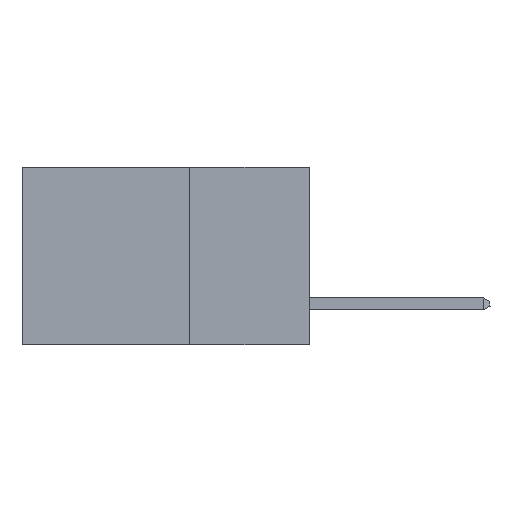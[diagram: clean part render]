
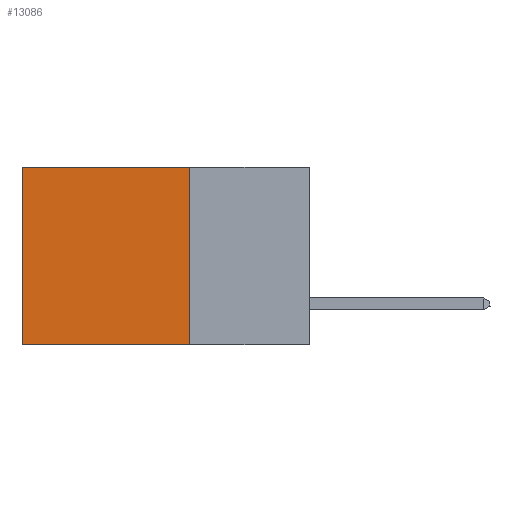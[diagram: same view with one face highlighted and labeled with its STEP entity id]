
A CAD part, left-side view. The second image highlights one B-rep face of the part: STEP entity #13086.
In plain terms, the highlighted planar face has unit normal (-1, 0, 0).
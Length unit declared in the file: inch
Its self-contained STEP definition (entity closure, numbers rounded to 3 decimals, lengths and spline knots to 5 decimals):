
#238 = VERTEX_POINT ( 'NONE', #27249 ) ;
#965 = CARTESIAN_POINT ( 'NONE',  ( 0.2875, 0.25, -0.37 ) ) ;
#1485 = VERTEX_POINT ( 'NONE', #13340 ) ;
#1870 = FACE_OUTER_BOUND ( 'NONE', #26713, .T. ) ;
#3059 = PLANE ( 'NONE',  #14644 ) ;
#4616 = LINE ( 'NONE', #22239, #10946 ) ;
#7609 = DIRECTION ( 'NONE',  ( 0., 1., 0. ) ) ;
#8184 = CARTESIAN_POINT ( 'NONE',  ( 0.2875, 0.6, -0.37 ) ) ;
#8716 = EDGE_CURVE ( 'NONE', #238, #26380, #4616, .T. ) ;
#10644 = CARTESIAN_POINT ( 'NONE',  ( 0.2875, 0.25, -0.37 ) ) ;
#10946 = VECTOR ( 'NONE', #24400, 39.37008 ) ;
#12156 = VECTOR ( 'NONE', #7609, 39.37008 ) ;
#13086 = ADVANCED_FACE ( 'NONE', ( #1870 ), #3059, .F. ) ;
#13340 = CARTESIAN_POINT ( 'NONE',  ( 0.2875, 0.6, 0. ) ) ;
#14644 = AXIS2_PLACEMENT_3D ( 'NONE', #20826, #16453, #18583 ) ;
#16453 = DIRECTION ( 'NONE',  ( 1., 0., 0. ) ) ;
#16570 = EDGE_CURVE ( 'NONE', #238, #1485, #28032, .T. ) ;
#16613 = EDGE_CURVE ( 'NONE', #1485, #22886, #25552, .T. ) ;
#17371 = DIRECTION ( 'NONE',  ( 0., 0., -1. ) ) ;
#17514 = VECTOR ( 'NONE', #28062, 39.37008 ) ;
#18132 = LINE ( 'NONE', #965, #12156 ) ;
#18583 = DIRECTION ( 'NONE',  ( 0., 0., -1. ) ) ;
#19599 = VECTOR ( 'NONE', #17371, 39.37008 ) ;
#20826 = CARTESIAN_POINT ( 'NONE',  ( 0.2875, 0.25, 0. ) ) ;
#21624 = CARTESIAN_POINT ( 'NONE',  ( 0.2875, 0.6, 0. ) ) ;
#22239 = CARTESIAN_POINT ( 'NONE',  ( 0.2875, 0.25, 0. ) ) ;
#22785 = ORIENTED_EDGE ( 'NONE', *, *, #25533, .F. ) ;
#22886 = VERTEX_POINT ( 'NONE', #8184 ) ;
#24400 = DIRECTION ( 'NONE',  ( 0., 0., -1. ) ) ;
#25533 = EDGE_CURVE ( 'NONE', #26380, #22886, #18132, .T. ) ;
#25552 = LINE ( 'NONE', #21624, #19599 ) ;
#26161 = CARTESIAN_POINT ( 'NONE',  ( 0.2875, 0.25, 0. ) ) ;
#26380 = VERTEX_POINT ( 'NONE', #10644 ) ;
#26713 = EDGE_LOOP ( 'NONE', ( #28991, #22785, #27672, #27090 ) ) ;
#27090 = ORIENTED_EDGE ( 'NONE', *, *, #16570, .T. ) ;
#27249 = CARTESIAN_POINT ( 'NONE',  ( 0.2875, 0.25, 0. ) ) ;
#27672 = ORIENTED_EDGE ( 'NONE', *, *, #8716, .F. ) ;
#28032 = LINE ( 'NONE', #26161, #17514 ) ;
#28062 = DIRECTION ( 'NONE',  ( 0., 1., 0. ) ) ;
#28991 = ORIENTED_EDGE ( 'NONE', *, *, #16613, .T. ) ;
